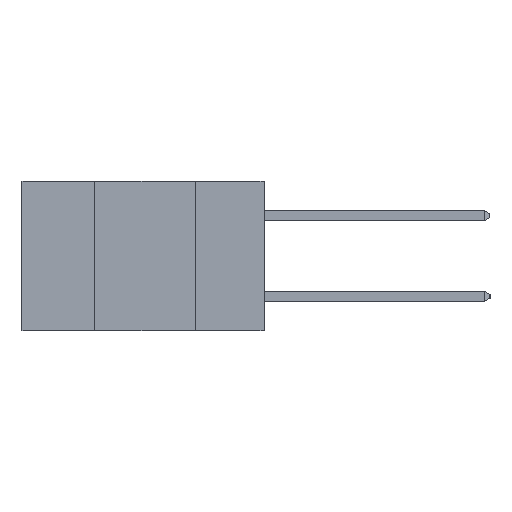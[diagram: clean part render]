
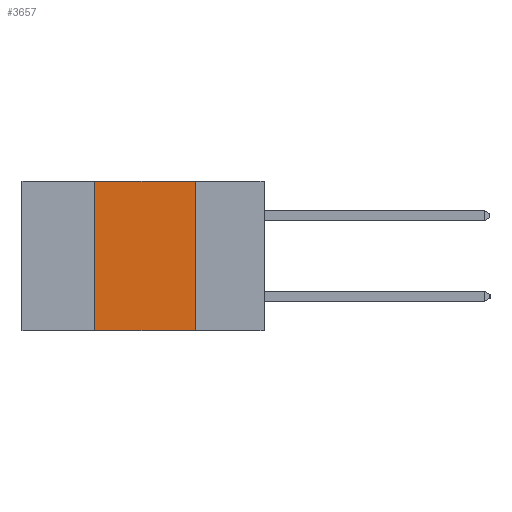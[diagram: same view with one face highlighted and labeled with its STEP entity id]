
A CAD part, left-side view. The second image highlights one B-rep face of the part: STEP entity #3657.
In plain terms, the highlighted planar face has unit normal (-1, 0, 0).
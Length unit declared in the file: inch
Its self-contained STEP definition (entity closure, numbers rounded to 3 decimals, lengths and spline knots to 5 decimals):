
#25 = CARTESIAN_POINT ( 'NONE',  ( 0., 0.17, 0. ) ) ;
#362 = PLANE ( 'NONE',  #2529 ) ;
#497 = ORIENTED_EDGE ( 'NONE', *, *, #5850, .F. ) ;
#1032 = VECTOR ( 'NONE', #5948, 39.37008 ) ;
#2529 = AXIS2_PLACEMENT_3D ( 'NONE', #2580, #9699, #3633 ) ;
#2580 = CARTESIAN_POINT ( 'NONE',  ( 0., 0.6, 0. ) ) ;
#2839 = CARTESIAN_POINT ( 'NONE',  ( 0., 0.42, -0.37 ) ) ;
#3022 = ORIENTED_EDGE ( 'NONE', *, *, #7265, .F. ) ;
#3541 = VECTOR ( 'NONE', #12156, 39.37008 ) ;
#3633 = DIRECTION ( 'NONE',  ( 0., 0., -1. ) ) ;
#3657 = ADVANCED_FACE ( 'NONE', ( #4550 ), #362, .F. ) ;
#3822 = VECTOR ( 'NONE', #6424, 39.37008 ) ;
#4067 = CARTESIAN_POINT ( 'NONE',  ( 0., 0.42, 0. ) ) ;
#4141 = LINE ( 'NONE', #12168, #3822 ) ;
#4467 = EDGE_CURVE ( 'NONE', #10735, #7861, #11334, .T. ) ;
#4550 = FACE_OUTER_BOUND ( 'NONE', #9953, .T. ) ;
#5175 = EDGE_CURVE ( 'NONE', #10735, #9391, #8661, .T. ) ;
#5788 = DIRECTION ( 'NONE',  ( 0., -1., 0. ) ) ;
#5821 = VECTOR ( 'NONE', #5788, 39.37008 ) ;
#5850 = EDGE_CURVE ( 'NONE', #9391, #7914, #6286, .T. ) ;
#5948 = DIRECTION ( 'NONE',  ( 0., 0., 1. ) ) ;
#6093 = ORIENTED_EDGE ( 'NONE', *, *, #5175, .F. ) ;
#6286 = LINE ( 'NONE', #8438, #3541 ) ;
#6424 = DIRECTION ( 'NONE',  ( 0., 0., -1. ) ) ;
#7265 = EDGE_CURVE ( 'NONE', #7914, #7861, #4141, .T. ) ;
#7861 = VERTEX_POINT ( 'NONE', #11161 ) ;
#7914 = VERTEX_POINT ( 'NONE', #25 ) ;
#8438 = CARTESIAN_POINT ( 'NONE',  ( 0., 0.6, 0. ) ) ;
#8661 = LINE ( 'NONE', #2839, #1032 ) ;
#8755 = CARTESIAN_POINT ( 'NONE',  ( 0., 0.6, -0.37 ) ) ;
#8789 = ORIENTED_EDGE ( 'NONE', *, *, #4467, .T. ) ;
#9391 = VERTEX_POINT ( 'NONE', #4067 ) ;
#9699 = DIRECTION ( 'NONE',  ( 1., 0., 0. ) ) ;
#9953 = EDGE_LOOP ( 'NONE', ( #3022, #497, #6093, #8789 ) ) ;
#10735 = VERTEX_POINT ( 'NONE', #12916 ) ;
#11161 = CARTESIAN_POINT ( 'NONE',  ( 0., 0.17, -0.37 ) ) ;
#11334 = LINE ( 'NONE', #8755, #5821 ) ;
#12156 = DIRECTION ( 'NONE',  ( 0., -1., 0. ) ) ;
#12168 = CARTESIAN_POINT ( 'NONE',  ( 0., 0.17, -0.37 ) ) ;
#12916 = CARTESIAN_POINT ( 'NONE',  ( 0., 0.42, -0.37 ) ) ;
